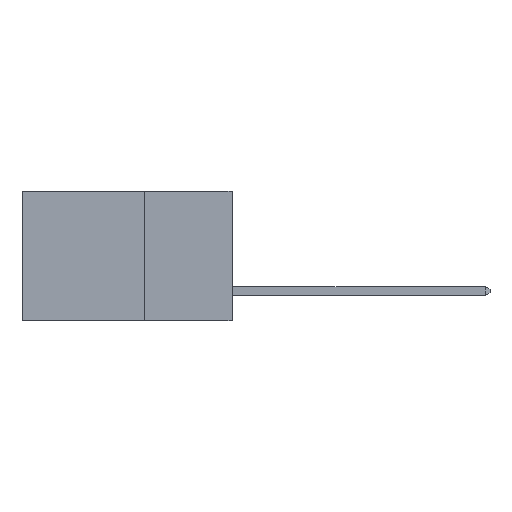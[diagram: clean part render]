
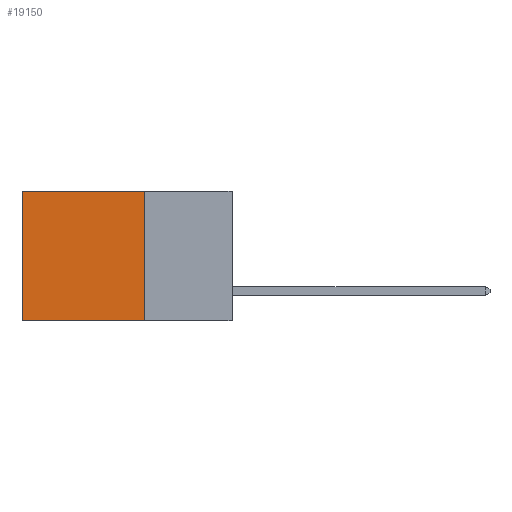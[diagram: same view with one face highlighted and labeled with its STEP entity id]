
A CAD part, left-side view. The second image highlights one B-rep face of the part: STEP entity #19150.
In plain terms, the highlighted planar face has unit normal (-1, 0, 0).
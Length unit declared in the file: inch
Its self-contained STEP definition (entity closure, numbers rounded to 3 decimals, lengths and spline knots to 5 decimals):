
#128 = ORIENTED_EDGE ( 'NONE', *, *, #6147, .F. ) ;
#423 = LINE ( 'NONE', #15741, #18191 ) ;
#926 = DIRECTION ( 'NONE',  ( 0., 0., -1. ) ) ;
#2257 = LINE ( 'NONE', #17412, #18920 ) ;
#2902 = VERTEX_POINT ( 'NONE', #16624 ) ;
#3403 = VECTOR ( 'NONE', #926, 39.37008 ) ;
#3910 = VERTEX_POINT ( 'NONE', #4149 ) ;
#4149 = CARTESIAN_POINT ( 'NONE',  ( 0.2875, 0.6, 0. ) ) ;
#5667 = DIRECTION ( 'NONE',  ( 0., 1., 0. ) ) ;
#6147 = EDGE_CURVE ( 'NONE', #2902, #8051, #423, .T. ) ;
#6682 = CARTESIAN_POINT ( 'NONE',  ( 0.2875, 0.25, 0. ) ) ;
#6712 = EDGE_CURVE ( 'NONE', #3910, #8051, #2257, .T. ) ;
#7402 = DIRECTION ( 'NONE',  ( 0., 0., -1. ) ) ;
#7582 = CARTESIAN_POINT ( 'NONE',  ( 0.2875, 0.25, 0. ) ) ;
#8004 = DIRECTION ( 'NONE',  ( 1., 0., 0. ) ) ;
#8051 = VERTEX_POINT ( 'NONE', #19128 ) ;
#9320 = ORIENTED_EDGE ( 'NONE', *, *, #19545, .T. ) ;
#12368 = LINE ( 'NONE', #7582, #3403 ) ;
#12439 = CARTESIAN_POINT ( 'NONE',  ( 0.2875, 0.25, 0. ) ) ;
#12591 = EDGE_CURVE ( 'NONE', #21085, #2902, #12368, .T. ) ;
#12761 = AXIS2_PLACEMENT_3D ( 'NONE', #14637, #8004, #19599 ) ;
#12851 = EDGE_LOOP ( 'NONE', ( #16831, #128, #19589, #9320 ) ) ;
#14637 = CARTESIAN_POINT ( 'NONE',  ( 0.2875, 0.25, 0. ) ) ;
#15360 = LINE ( 'NONE', #12439, #19668 ) ;
#15741 = CARTESIAN_POINT ( 'NONE',  ( 0.2875, 0.25, -0.37 ) ) ;
#16624 = CARTESIAN_POINT ( 'NONE',  ( 0.2875, 0.25, -0.37 ) ) ;
#16831 = ORIENTED_EDGE ( 'NONE', *, *, #6712, .T. ) ;
#17412 = CARTESIAN_POINT ( 'NONE',  ( 0.2875, 0.6, 0. ) ) ;
#17998 = PLANE ( 'NONE',  #12761 ) ;
#18191 = VECTOR ( 'NONE', #5667, 39.37008 ) ;
#18920 = VECTOR ( 'NONE', #7402, 39.37008 ) ;
#19128 = CARTESIAN_POINT ( 'NONE',  ( 0.2875, 0.6, -0.37 ) ) ;
#19150 = ADVANCED_FACE ( 'NONE', ( #19180 ), #17998, .F. ) ;
#19180 = FACE_OUTER_BOUND ( 'NONE', #12851, .T. ) ;
#19545 = EDGE_CURVE ( 'NONE', #21085, #3910, #15360, .T. ) ;
#19589 = ORIENTED_EDGE ( 'NONE', *, *, #12591, .F. ) ;
#19599 = DIRECTION ( 'NONE',  ( 0., 0., -1. ) ) ;
#19668 = VECTOR ( 'NONE', #20599, 39.37008 ) ;
#20599 = DIRECTION ( 'NONE',  ( 0., 1., 0. ) ) ;
#21085 = VERTEX_POINT ( 'NONE', #6682 ) ;
